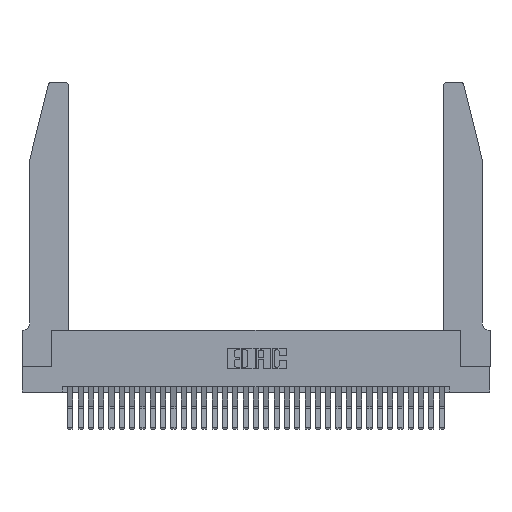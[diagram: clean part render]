
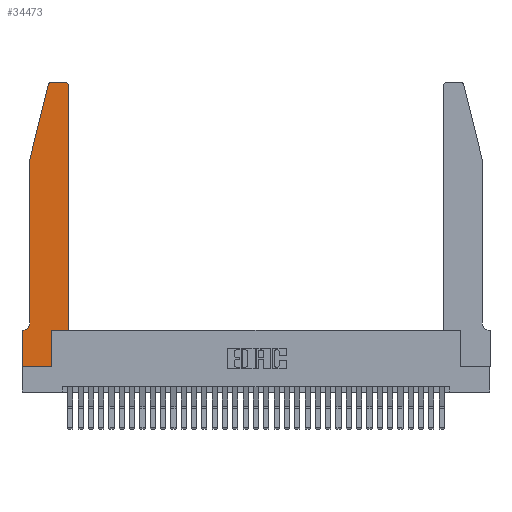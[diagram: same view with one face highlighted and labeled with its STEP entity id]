
A CAD part, top view. The second image highlights one B-rep face of the part: STEP entity #34473.
In plain terms, the highlighted planar face has unit normal (0, 0, 1).
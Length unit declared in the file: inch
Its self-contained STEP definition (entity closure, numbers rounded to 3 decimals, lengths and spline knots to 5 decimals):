
#248 = ORIENTED_EDGE ( 'NONE', *, *, #30124, .T. ) ;
#290 = CIRCLE ( 'NONE', #23841, 0.07 ) ;
#318 = CARTESIAN_POINT ( 'NONE',  ( 0.0755, 0.42, 0.37 ) ) ;
#860 = VECTOR ( 'NONE', #31409, 39.37008 ) ;
#918 = ORIENTED_EDGE ( 'NONE', *, *, #10100, .T. ) ;
#1128 = LINE ( 'NONE', #29292, #15468 ) ;
#1834 = AXIS2_PLACEMENT_3D ( 'NONE', #25484, #9433, #28138 ) ;
#1946 = DIRECTION ( 'NONE',  ( -1., 0., 0. ) ) ;
#2243 = CARTESIAN_POINT ( 'NONE',  ( 0.4505, 0.35, 0.37 ) ) ;
#2485 = EDGE_CURVE ( 'NONE', #15784, #17213, #6676, .T. ) ;
#2803 = ORIENTED_EDGE ( 'NONE', *, *, #9431, .T. ) ;
#3575 = LINE ( 'NONE', #29288, #30351 ) ;
#3658 = CARTESIAN_POINT ( 'NONE',  ( 0., 0.35, 0.37 ) ) ;
#4588 = CARTESIAN_POINT ( 'NONE',  ( 0.0755, 2., 0.37 ) ) ;
#4930 = VERTEX_POINT ( 'NONE', #23716 ) ;
#4951 = DIRECTION ( 'NONE',  ( 1., 0., 0. ) ) ;
#4973 = CARTESIAN_POINT ( 'NONE',  ( 0.4505, 2.72, 0.37 ) ) ;
#5580 = CIRCLE ( 'NONE', #1834, 0.03 ) ;
#5837 = VECTOR ( 'NONE', #31994, 39.37008 ) ;
#5927 = VECTOR ( 'NONE', #24648, 39.37008 ) ;
#6539 = ORIENTED_EDGE ( 'NONE', *, *, #16596, .T. ) ;
#6676 = LINE ( 'NONE', #16126, #5837 ) ;
#6859 = LINE ( 'NONE', #2243, #34376 ) ;
#7219 = VECTOR ( 'NONE', #15430, 39.37008 ) ;
#7313 = VERTEX_POINT ( 'NONE', #16532 ) ;
#8581 = CARTESIAN_POINT ( 'NONE',  ( 0.4505, 0.35, 0.37 ) ) ;
#9087 = DIRECTION ( 'NONE',  ( 1., 0., 0. ) ) ;
#9137 = ORIENTED_EDGE ( 'NONE', *, *, #14602, .T. ) ;
#9431 = EDGE_CURVE ( 'NONE', #17213, #19634, #21542, .T. ) ;
#9433 = DIRECTION ( 'NONE',  ( 0., 0., 1. ) ) ;
#10013 = VERTEX_POINT ( 'NONE', #28203 ) ;
#10100 = EDGE_CURVE ( 'NONE', #30868, #10013, #290, .T. ) ;
#10567 = CARTESIAN_POINT ( 'NONE',  ( 0.25487, 2.72718, 0.37 ) ) ;
#10756 = CARTESIAN_POINT ( 'NONE',  ( 0.2865, 0., 0.37 ) ) ;
#11024 = CARTESIAN_POINT ( 'NONE',  ( 0., 0., 0.37 ) ) ;
#11255 = ORIENTED_EDGE ( 'NONE', *, *, #2485, .T. ) ;
#11314 = CARTESIAN_POINT ( 'NONE',  ( 0.0755, 2., 0.37 ) ) ;
#12447 = ORIENTED_EDGE ( 'NONE', *, *, #26523, .T. ) ;
#12466 = EDGE_LOOP ( 'NONE', ( #29798, #20331, #9137, #248, #918, #12447, #11255, #2803, #33422, #6539, #14855, #24696 ) ) ;
#14420 = PLANE ( 'NONE',  #32933 ) ;
#14602 = EDGE_CURVE ( 'NONE', #14733, #32506, #21473, .T. ) ;
#14708 = VECTOR ( 'NONE', #15445, 39.37008 ) ;
#14733 = VERTEX_POINT ( 'NONE', #10567 ) ;
#14855 = ORIENTED_EDGE ( 'NONE', *, *, #28805, .T. ) ;
#15255 = CARTESIAN_POINT ( 'NONE',  ( 0.4205, 2.72, 0.37 ) ) ;
#15321 = CARTESIAN_POINT ( 'NONE',  ( 0., 0., 0.37 ) ) ;
#15366 = CARTESIAN_POINT ( 'NONE',  ( 0.2865, 0.35, 0.37 ) ) ;
#15430 = DIRECTION ( 'NONE',  ( 1., 0., 0. ) ) ;
#15445 = DIRECTION ( 'NONE',  ( 0., -1., 0. ) ) ;
#15468 = VECTOR ( 'NONE', #21295, 39.37008 ) ;
#15784 = VERTEX_POINT ( 'NONE', #25170 ) ;
#16126 = CARTESIAN_POINT ( 'NONE',  ( 0., 0., 0.37 ) ) ;
#16532 = CARTESIAN_POINT ( 'NONE',  ( 0.4505, 0.35, 0.37 ) ) ;
#16596 = EDGE_CURVE ( 'NONE', #17656, #7313, #6859, .T. ) ;
#17213 = VERTEX_POINT ( 'NONE', #11024 ) ;
#17656 = VERTEX_POINT ( 'NONE', #15366 ) ;
#17924 = DIRECTION ( 'NONE',  ( 1., 0., 0. ) ) ;
#17945 = CARTESIAN_POINT ( 'NONE',  ( 0.4205, 2.75, 0.37 ) ) ;
#18061 = DIRECTION ( 'NONE',  ( 0., 0., -1. ) ) ;
#18165 = CARTESIAN_POINT ( 'NONE',  ( 0.2605, 2.75, 0.37 ) ) ;
#18451 = LINE ( 'NONE', #18165, #32538 ) ;
#19393 = LINE ( 'NONE', #8581, #5927 ) ;
#19532 = VERTEX_POINT ( 'NONE', #4973 ) ;
#19634 = VERTEX_POINT ( 'NONE', #10756 ) ;
#20169 = EDGE_CURVE ( 'NONE', #19634, #17656, #1128, .T. ) ;
#20331 = ORIENTED_EDGE ( 'NONE', *, *, #34554, .T. ) ;
#20786 = CARTESIAN_POINT ( 'NONE',  ( 0.0755, 2., 0.37 ) ) ;
#20865 = DIRECTION ( 'NONE',  ( -1., 0., 0. ) ) ;
#21212 = AXIS2_PLACEMENT_3D ( 'NONE', #15255, #33784, #17924 ) ;
#21295 = DIRECTION ( 'NONE',  ( 0., 1., 0. ) ) ;
#21473 = LINE ( 'NONE', #20786, #860 ) ;
#21542 = LINE ( 'NONE', #15321, #7219 ) ;
#21830 = LINE ( 'NONE', #4588, #14708 ) ;
#23716 = CARTESIAN_POINT ( 'NONE',  ( 0.284, 2.75, 0.37 ) ) ;
#23841 = AXIS2_PLACEMENT_3D ( 'NONE', #33916, #18061, #1946 ) ;
#23847 = EDGE_CURVE ( 'NONE', #27255, #4930, #18451, .T. ) ;
#24648 = DIRECTION ( 'NONE',  ( 0., 1., 0. ) ) ;
#24696 = ORIENTED_EDGE ( 'NONE', *, *, #33990, .T. ) ;
#25140 = DIRECTION ( 'NONE',  ( 0., 0., 1. ) ) ;
#25170 = CARTESIAN_POINT ( 'NONE',  ( 0., 0.35, 0.37 ) ) ;
#25484 = CARTESIAN_POINT ( 'NONE',  ( 0.284, 2.72, 0.37 ) ) ;
#26523 = EDGE_CURVE ( 'NONE', #10013, #15784, #3575, .T. ) ;
#27255 = VERTEX_POINT ( 'NONE', #17945 ) ;
#28138 = DIRECTION ( 'NONE',  ( 1., 0., 0. ) ) ;
#28203 = CARTESIAN_POINT ( 'NONE',  ( 0.0055, 0.35, 0.37 ) ) ;
#28611 = FACE_OUTER_BOUND ( 'NONE', #12466, .T. ) ;
#28805 = EDGE_CURVE ( 'NONE', #7313, #19532, #19393, .T. ) ;
#29288 = CARTESIAN_POINT ( 'NONE',  ( 0.0755, 0.35, 0.37 ) ) ;
#29292 = CARTESIAN_POINT ( 'NONE',  ( 0.2865, 0.35, 0.37 ) ) ;
#29479 = CIRCLE ( 'NONE', #21212, 0.03 ) ;
#29798 = ORIENTED_EDGE ( 'NONE', *, *, #23847, .T. ) ;
#30124 = EDGE_CURVE ( 'NONE', #32506, #30868, #21830, .T. ) ;
#30351 = VECTOR ( 'NONE', #31905, 39.37008 ) ;
#30868 = VERTEX_POINT ( 'NONE', #318 ) ;
#31409 = DIRECTION ( 'NONE',  ( -0.239, -0.971, 0. ) ) ;
#31905 = DIRECTION ( 'NONE',  ( -1., 0., 0. ) ) ;
#31994 = DIRECTION ( 'NONE',  ( 0., -1., 0. ) ) ;
#32506 = VERTEX_POINT ( 'NONE', #11314 ) ;
#32538 = VECTOR ( 'NONE', #20865, 39.37008 ) ;
#32933 = AXIS2_PLACEMENT_3D ( 'NONE', #3658, #25140, #9087 ) ;
#33422 = ORIENTED_EDGE ( 'NONE', *, *, #20169, .T. ) ;
#33784 = DIRECTION ( 'NONE',  ( 0., 0., 1. ) ) ;
#33916 = CARTESIAN_POINT ( 'NONE',  ( 0.0055, 0.42, 0.37 ) ) ;
#33990 = EDGE_CURVE ( 'NONE', #19532, #27255, #29479, .T. ) ;
#34376 = VECTOR ( 'NONE', #4951, 39.37008 ) ;
#34473 = ADVANCED_FACE ( 'NONE', ( #28611 ), #14420, .T. ) ;
#34554 = EDGE_CURVE ( 'NONE', #4930, #14733, #5580, .T. ) ;
